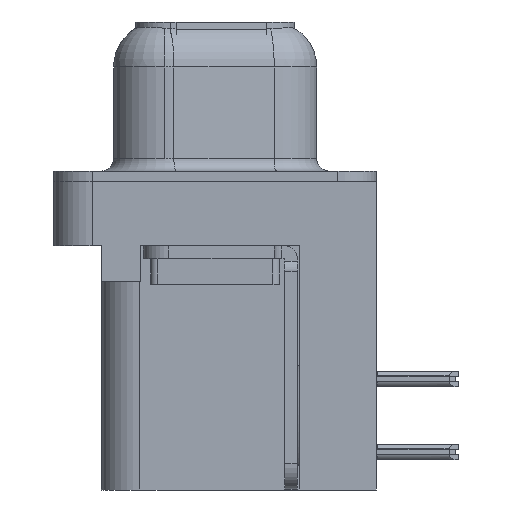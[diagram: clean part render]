
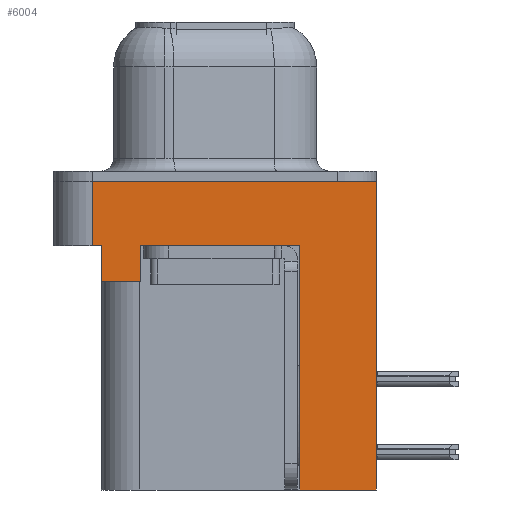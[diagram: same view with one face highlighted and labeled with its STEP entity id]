
A CAD part, left-side view. The second image highlights one B-rep face of the part: STEP entity #6004.
In plain terms, the highlighted planar face has unit normal (-1, 0, 0).
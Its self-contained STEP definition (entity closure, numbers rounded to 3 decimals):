
#218 = LINE ( 'NONE', #20145, #14459 ) ;
#900 = DIRECTION ( 'NONE',  ( 0., 1., 0. ) ) ;
#1020 = CARTESIAN_POINT ( 'NONE',  ( -2.91, 4.425, -2.5 ) ) ;
#1251 = CARTESIAN_POINT ( 'NONE',  ( -2.91, 4.775, -2.5 ) ) ;
#2396 = PLANE ( 'NONE',  #17313 ) ;
#2854 = EDGE_CURVE ( 'NONE', #8888, #11045, #35374, .T. ) ;
#2902 = CARTESIAN_POINT ( 'NONE',  ( -2.91, -6.275, -12. ) ) ;
#3136 = LINE ( 'NONE', #18182, #34680 ) ;
#3377 = CARTESIAN_POINT ( 'NONE',  ( -2.91, 2.895, -3.9 ) ) ;
#3504 = CARTESIAN_POINT ( 'NONE',  ( -2.91, 4.775, 0. ) ) ;
#3616 = DIRECTION ( 'NONE',  ( 0., -1., 0. ) ) ;
#4579 = EDGE_CURVE ( 'NONE', #29717, #36725, #37188, .T. ) ;
#5913 = EDGE_CURVE ( 'NONE', #13958, #33569, #20299, .T. ) ;
#6004 = ADVANCED_FACE ( 'NONE', ( #33465 ), #2396, .T. ) ;
#6329 = CARTESIAN_POINT ( 'NONE',  ( -2.91, -3.295, -2.5 ) ) ;
#6505 = ORIENTED_EDGE ( 'NONE', *, *, #6779, .F. ) ;
#6596 = LINE ( 'NONE', #20601, #9820 ) ;
#6753 = CARTESIAN_POINT ( 'NONE',  ( -2.91, 4.425, -3.9 ) ) ;
#6779 = EDGE_CURVE ( 'NONE', #7350, #15454, #36166, .T. ) ;
#7001 = CARTESIAN_POINT ( 'NONE',  ( -2.91, -6.275, 0. ) ) ;
#7350 = VERTEX_POINT ( 'NONE', #2902 ) ;
#8362 = ORIENTED_EDGE ( 'NONE', *, *, #21480, .F. ) ;
#8888 = VERTEX_POINT ( 'NONE', #33564 ) ;
#9777 = VECTOR ( 'NONE', #18489, 1000. ) ;
#9820 = VECTOR ( 'NONE', #32121, 1000. ) ;
#10481 = CARTESIAN_POINT ( 'NONE',  ( -2.91, 2.895, -2.5 ) ) ;
#10573 = VECTOR ( 'NONE', #11892, 1000. ) ;
#11045 = VERTEX_POINT ( 'NONE', #10481 ) ;
#11126 = DIRECTION ( 'NONE',  ( 0., -1., 0. ) ) ;
#11241 = DIRECTION ( 'NONE',  ( -1., 0., 0. ) ) ;
#11892 = DIRECTION ( 'NONE',  ( 0., 1., 0. ) ) ;
#13518 = EDGE_CURVE ( 'NONE', #13958, #36725, #218, .T. ) ;
#13561 = ORIENTED_EDGE ( 'NONE', *, *, #14788, .T. ) ;
#13866 = ORIENTED_EDGE ( 'NONE', *, *, #2854, .T. ) ;
#13958 = VERTEX_POINT ( 'NONE', #16628 ) ;
#14385 = LINE ( 'NONE', #18614, #9777 ) ;
#14459 = VECTOR ( 'NONE', #11126, 1000. ) ;
#14788 = EDGE_CURVE ( 'NONE', #11045, #25471, #14385, .T. ) ;
#14865 = ORIENTED_EDGE ( 'NONE', *, *, #5913, .F. ) ;
#14897 = VECTOR ( 'NONE', #900, 1000. ) ;
#15454 = VERTEX_POINT ( 'NONE', #32850 ) ;
#15711 = CARTESIAN_POINT ( 'NONE',  ( -2.91, -6.275, 0. ) ) ;
#16628 = CARTESIAN_POINT ( 'NONE',  ( -2.91, 4.775, -2.5 ) ) ;
#17313 = AXIS2_PLACEMENT_3D ( 'NONE', #28753, #11241, #31645 ) ;
#17614 = ORIENTED_EDGE ( 'NONE', *, *, #4579, .F. ) ;
#18182 = CARTESIAN_POINT ( 'NONE',  ( -2.91, -3.295, -12. ) ) ;
#18489 = DIRECTION ( 'NONE',  ( 0., -1., 0. ) ) ;
#18614 = CARTESIAN_POINT ( 'NONE',  ( -2.91, -6.275, -2.5 ) ) ;
#19110 = LINE ( 'NONE', #6753, #14897 ) ;
#19137 = EDGE_CURVE ( 'NONE', #8888, #29717, #19110, .T. ) ;
#19843 = ORIENTED_EDGE ( 'NONE', *, *, #26421, .T. ) ;
#20145 = CARTESIAN_POINT ( 'NONE',  ( -2.91, -6.275, -2.5 ) ) ;
#20299 = LINE ( 'NONE', #1251, #22157 ) ;
#20601 = CARTESIAN_POINT ( 'NONE',  ( -2.91, -6.275, -2.5 ) ) ;
#20680 = LINE ( 'NONE', #15711, #26163 ) ;
#21480 = EDGE_CURVE ( 'NONE', #15454, #25471, #3136, .T. ) ;
#21808 = DIRECTION ( 'NONE',  ( 0., 0., 1. ) ) ;
#22157 = VECTOR ( 'NONE', #21808, 1000. ) ;
#25349 = CARTESIAN_POINT ( 'NONE',  ( -2.91, 4.425, -3.9 ) ) ;
#25471 = VERTEX_POINT ( 'NONE', #6329 ) ;
#26163 = VECTOR ( 'NONE', #3616, 1000. ) ;
#26421 = EDGE_CURVE ( 'NONE', #7350, #34256, #6596, .T. ) ;
#28079 = VECTOR ( 'NONE', #30301, 1000. ) ;
#28164 = ORIENTED_EDGE ( 'NONE', *, *, #19137, .F. ) ;
#28753 = CARTESIAN_POINT ( 'NONE',  ( -2.91, -6.275, -2.5 ) ) ;
#28898 = CARTESIAN_POINT ( 'NONE',  ( -2.91, -3.295, -12. ) ) ;
#29435 = EDGE_CURVE ( 'NONE', #33569, #34256, #20680, .T. ) ;
#29536 = EDGE_LOOP ( 'NONE', ( #32298, #14865, #30847, #17614, #28164, #13866, #13561, #8362, #6505, #19843 ) ) ;
#29717 = VERTEX_POINT ( 'NONE', #25349 ) ;
#29885 = DIRECTION ( 'NONE',  ( 0., 0., 1. ) ) ;
#30301 = DIRECTION ( 'NONE',  ( 0., 0., 1. ) ) ;
#30847 = ORIENTED_EDGE ( 'NONE', *, *, #13518, .T. ) ;
#31645 = DIRECTION ( 'NONE',  ( 0., 0., 1. ) ) ;
#32121 = DIRECTION ( 'NONE',  ( 0., 0., 1. ) ) ;
#32298 = ORIENTED_EDGE ( 'NONE', *, *, #29435, .F. ) ;
#32813 = CARTESIAN_POINT ( 'NONE',  ( -2.91, 4.425, -3.9 ) ) ;
#32850 = CARTESIAN_POINT ( 'NONE',  ( -2.91, -3.295, -12. ) ) ;
#33465 = FACE_OUTER_BOUND ( 'NONE', #29536, .T. ) ;
#33564 = CARTESIAN_POINT ( 'NONE',  ( -2.91, 2.895, -3.9 ) ) ;
#33569 = VERTEX_POINT ( 'NONE', #3504 ) ;
#34256 = VERTEX_POINT ( 'NONE', #7001 ) ;
#34446 = VECTOR ( 'NONE', #35610, 1000. ) ;
#34680 = VECTOR ( 'NONE', #29885, 1000. ) ;
#35374 = LINE ( 'NONE', #3377, #34446 ) ;
#35610 = DIRECTION ( 'NONE',  ( 0., 0., 1. ) ) ;
#36166 = LINE ( 'NONE', #28898, #10573 ) ;
#36725 = VERTEX_POINT ( 'NONE', #1020 ) ;
#37188 = LINE ( 'NONE', #32813, #28079 ) ;
